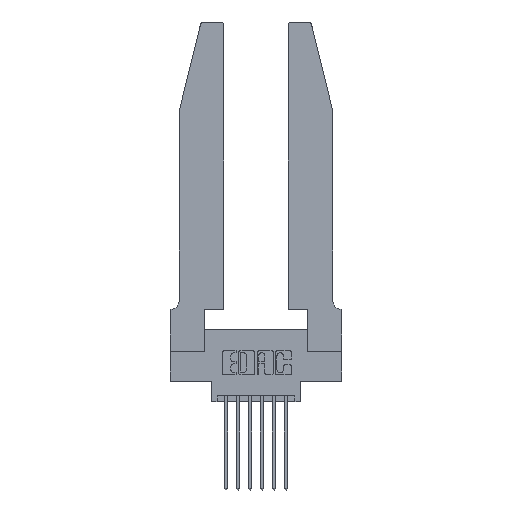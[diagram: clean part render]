
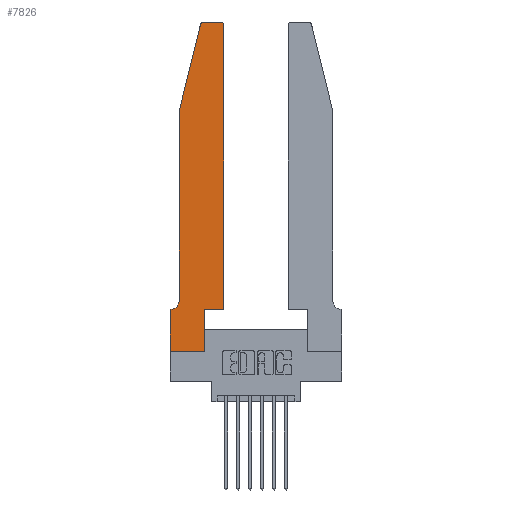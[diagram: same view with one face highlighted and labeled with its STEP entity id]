
A CAD part, top view. The second image highlights one B-rep face of the part: STEP entity #7826.
In plain terms, the highlighted planar face has unit normal (0, 0, 1).
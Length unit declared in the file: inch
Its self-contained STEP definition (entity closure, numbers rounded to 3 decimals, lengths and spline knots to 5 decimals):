
#92 = CARTESIAN_POINT ( 'NONE',  ( 0., 0., 0.37 ) ) ;
#100 = EDGE_CURVE ( 'NONE', #8857, #7002, #6327, .T. ) ;
#378 = EDGE_CURVE ( 'NONE', #7002, #486, #8804, .T. ) ;
#486 = VERTEX_POINT ( 'NONE', #6536 ) ;
#666 = EDGE_CURVE ( 'NONE', #1194, #7047, #14173, .T. ) ;
#744 = DIRECTION ( 'NONE',  ( 1., 0., 0. ) ) ;
#880 = ORIENTED_EDGE ( 'NONE', *, *, #10708, .T. ) ;
#1045 = ORIENTED_EDGE ( 'NONE', *, *, #8470, .T. ) ;
#1194 = VERTEX_POINT ( 'NONE', #11615 ) ;
#1632 = VERTEX_POINT ( 'NONE', #6832 ) ;
#1649 = DIRECTION ( 'NONE',  ( -1., 0., 0. ) ) ;
#1948 = DIRECTION ( 'NONE',  ( 0., 1., 0. ) ) ;
#1957 = VECTOR ( 'NONE', #744, 39.37008 ) ;
#2088 = CARTESIAN_POINT ( 'NONE',  ( 0.0055, 0.42, 0.37 ) ) ;
#2094 = ORIENTED_EDGE ( 'NONE', *, *, #100, .T. ) ;
#2210 = FACE_OUTER_BOUND ( 'NONE', #11139, .T. ) ;
#2467 = DIRECTION ( 'NONE',  ( 0., -1., 0. ) ) ;
#2602 = CARTESIAN_POINT ( 'NONE',  ( 0., 0.35, 0.37 ) ) ;
#2711 = LINE ( 'NONE', #8339, #5635 ) ;
#2821 = CARTESIAN_POINT ( 'NONE',  ( 0.2865, 0., 0.37 ) ) ;
#2852 = VECTOR ( 'NONE', #6102, 39.37008 ) ;
#3044 = CARTESIAN_POINT ( 'NONE',  ( 0.2865, 0.35, 0.37 ) ) ;
#3154 = EDGE_CURVE ( 'NONE', #5110, #1194, #5219, .T. ) ;
#3286 = CARTESIAN_POINT ( 'NONE',  ( 0.284, 2.75, 0.37 ) ) ;
#3502 = DIRECTION ( 'NONE',  ( 0., 0., 1. ) ) ;
#3598 = CIRCLE ( 'NONE', #11128, 0.03 ) ;
#3658 = DIRECTION ( 'NONE',  ( 0., 0., 1. ) ) ;
#3730 = LINE ( 'NONE', #7593, #12717 ) ;
#3742 = VERTEX_POINT ( 'NONE', #10978 ) ;
#3827 = AXIS2_PLACEMENT_3D ( 'NONE', #2602, #3658, #11532 ) ;
#3997 = CARTESIAN_POINT ( 'NONE',  ( 0.284, 2.72, 0.37 ) ) ;
#4086 = VECTOR ( 'NONE', #1948, 39.37008 ) ;
#4088 = VECTOR ( 'NONE', #2467, 39.37008 ) ;
#4197 = DIRECTION ( 'NONE',  ( 1., 0., 0. ) ) ;
#4347 = VERTEX_POINT ( 'NONE', #10219 ) ;
#4954 = CARTESIAN_POINT ( 'NONE',  ( 0.0055, 0.35, 0.37 ) ) ;
#5011 = ORIENTED_EDGE ( 'NONE', *, *, #378, .T. ) ;
#5110 = VERTEX_POINT ( 'NONE', #12687 ) ;
#5137 = DIRECTION ( 'NONE',  ( 1., 0., 0. ) ) ;
#5219 = LINE ( 'NONE', #10276, #1957 ) ;
#5368 = ORIENTED_EDGE ( 'NONE', *, *, #12758, .T. ) ;
#5635 = VECTOR ( 'NONE', #1649, 39.37008 ) ;
#5667 = EDGE_CURVE ( 'NONE', #486, #12838, #10461, .T. ) ;
#5907 = DIRECTION ( 'NONE',  ( 0., 0., -1. ) ) ;
#6049 = CARTESIAN_POINT ( 'NONE',  ( 0.0755, 2., 0.37 ) ) ;
#6102 = DIRECTION ( 'NONE',  ( -1., 0., 0. ) ) ;
#6327 = CIRCLE ( 'NONE', #10583, 0.07 ) ;
#6536 = CARTESIAN_POINT ( 'NONE',  ( 0., 0.35, 0.37 ) ) ;
#6592 = CARTESIAN_POINT ( 'NONE',  ( 0.0755, 2., 0.37 ) ) ;
#6832 = CARTESIAN_POINT ( 'NONE',  ( 0.0755, 2., 0.37 ) ) ;
#6980 = ORIENTED_EDGE ( 'NONE', *, *, #12664, .T. ) ;
#7002 = VERTEX_POINT ( 'NONE', #4954 ) ;
#7047 = VERTEX_POINT ( 'NONE', #9553 ) ;
#7205 = DIRECTION ( 'NONE',  ( 0., -1., 0. ) ) ;
#7343 = ORIENTED_EDGE ( 'NONE', *, *, #11130, .T. ) ;
#7593 = CARTESIAN_POINT ( 'NONE',  ( 0., 0., 0.37 ) ) ;
#7826 = ADVANCED_FACE ( 'NONE', ( #2210 ), #9300, .T. ) ;
#8339 = CARTESIAN_POINT ( 'NONE',  ( 0.2605, 2.75, 0.37 ) ) ;
#8377 = DIRECTION ( 'NONE',  ( 0., 1., 0. ) ) ;
#8391 = ORIENTED_EDGE ( 'NONE', *, *, #12185, .T. ) ;
#8470 = EDGE_CURVE ( 'NONE', #3742, #10113, #2711, .T. ) ;
#8496 = VERTEX_POINT ( 'NONE', #2821 ) ;
#8735 = ORIENTED_EDGE ( 'NONE', *, *, #3154, .T. ) ;
#8804 = LINE ( 'NONE', #12589, #2852 ) ;
#8857 = VERTEX_POINT ( 'NONE', #13400 ) ;
#8874 = LINE ( 'NONE', #6049, #11489 ) ;
#9300 = PLANE ( 'NONE',  #3827 ) ;
#9553 = CARTESIAN_POINT ( 'NONE',  ( 0.4505, 2.72, 0.37 ) ) ;
#9579 = VECTOR ( 'NONE', #11061, 39.37008 ) ;
#10113 = VERTEX_POINT ( 'NONE', #3286 ) ;
#10219 = CARTESIAN_POINT ( 'NONE',  ( 0.25487, 2.72718, 0.37 ) ) ;
#10258 = CARTESIAN_POINT ( 'NONE',  ( 0.4205, 2.72, 0.37 ) ) ;
#10276 = CARTESIAN_POINT ( 'NONE',  ( 0.4505, 0.35, 0.37 ) ) ;
#10319 = ORIENTED_EDGE ( 'NONE', *, *, #12561, .T. ) ;
#10455 = LINE ( 'NONE', #3044, #4086 ) ;
#10461 = LINE ( 'NONE', #92, #4088 ) ;
#10583 = AXIS2_PLACEMENT_3D ( 'NONE', #2088, #5907, #11721 ) ;
#10708 = EDGE_CURVE ( 'NONE', #7047, #3742, #3598, .T. ) ;
#10978 = CARTESIAN_POINT ( 'NONE',  ( 0.4205, 2.75, 0.37 ) ) ;
#11014 = ORIENTED_EDGE ( 'NONE', *, *, #5667, .T. ) ;
#11061 = DIRECTION ( 'NONE',  ( -0.239, -0.971, 0. ) ) ;
#11128 = AXIS2_PLACEMENT_3D ( 'NONE', #10258, #3502, #11366 ) ;
#11130 = EDGE_CURVE ( 'NONE', #4347, #1632, #12904, .T. ) ;
#11139 = EDGE_LOOP ( 'NONE', ( #1045, #6980, #7343, #10319, #2094, #5011, #11014, #5368, #8391, #8735, #12070, #880 ) ) ;
#11198 = CARTESIAN_POINT ( 'NONE',  ( 0., 0., 0.37 ) ) ;
#11366 = DIRECTION ( 'NONE',  ( 1., 0., 0. ) ) ;
#11489 = VECTOR ( 'NONE', #7205, 39.37008 ) ;
#11532 = DIRECTION ( 'NONE',  ( 1., 0., 0. ) ) ;
#11615 = CARTESIAN_POINT ( 'NONE',  ( 0.4505, 0.35, 0.37 ) ) ;
#11721 = DIRECTION ( 'NONE',  ( -1., 0., 0. ) ) ;
#11893 = DIRECTION ( 'NONE',  ( 0., 0., 1. ) ) ;
#11953 = CARTESIAN_POINT ( 'NONE',  ( 0.4505, 0.35, 0.37 ) ) ;
#12070 = ORIENTED_EDGE ( 'NONE', *, *, #666, .T. ) ;
#12185 = EDGE_CURVE ( 'NONE', #8496, #5110, #10455, .T. ) ;
#12448 = AXIS2_PLACEMENT_3D ( 'NONE', #3997, #11893, #5137 ) ;
#12561 = EDGE_CURVE ( 'NONE', #1632, #8857, #8874, .T. ) ;
#12589 = CARTESIAN_POINT ( 'NONE',  ( 0.0755, 0.35, 0.37 ) ) ;
#12664 = EDGE_CURVE ( 'NONE', #10113, #4347, #13399, .T. ) ;
#12687 = CARTESIAN_POINT ( 'NONE',  ( 0.2865, 0.35, 0.37 ) ) ;
#12717 = VECTOR ( 'NONE', #4197, 39.37008 ) ;
#12758 = EDGE_CURVE ( 'NONE', #12838, #8496, #3730, .T. ) ;
#12838 = VERTEX_POINT ( 'NONE', #11198 ) ;
#12904 = LINE ( 'NONE', #6592, #9579 ) ;
#13399 = CIRCLE ( 'NONE', #12448, 0.03 ) ;
#13400 = CARTESIAN_POINT ( 'NONE',  ( 0.0755, 0.42, 0.37 ) ) ;
#13833 = VECTOR ( 'NONE', #8377, 39.37008 ) ;
#14173 = LINE ( 'NONE', #11953, #13833 ) ;
